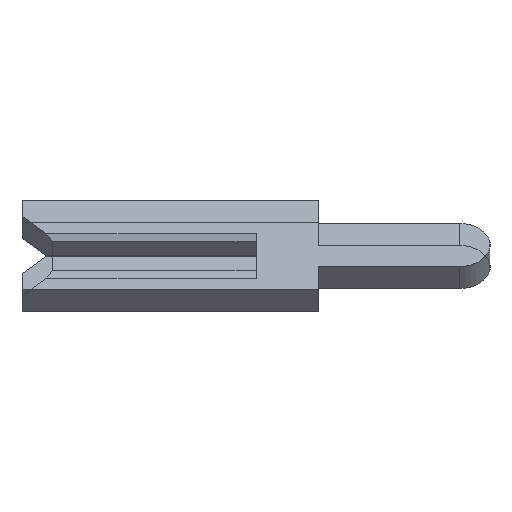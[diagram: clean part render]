
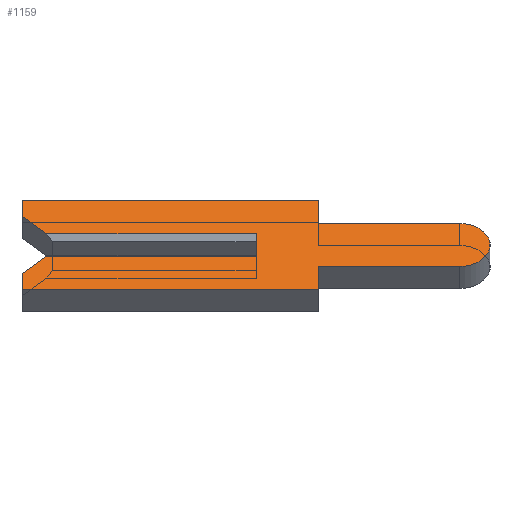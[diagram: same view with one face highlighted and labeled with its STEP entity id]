
A CAD part, left-side view. The second image highlights one B-rep face of the part: STEP entity #1159.
In plain terms, the highlighted face is planar.
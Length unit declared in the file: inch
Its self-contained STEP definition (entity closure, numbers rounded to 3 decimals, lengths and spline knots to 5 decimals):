
#26 = EDGE_CURVE ( 'NONE', #1658, #209, #2182, .T. ) ;
#27 = VERTEX_POINT ( 'NONE', #2498 ) ;
#85 = VECTOR ( 'NONE', #3154, 39.37008 ) ;
#199 = LINE ( 'NONE', #3491, #3130 ) ;
#203 = ORIENTED_EDGE ( 'NONE', *, *, #2566, .F. ) ;
#209 = VERTEX_POINT ( 'NONE', #977 ) ;
#218 = AXIS2_PLACEMENT_3D ( 'NONE', #1717, #3476, #2283 ) ;
#241 = LINE ( 'NONE', #670, #3102 ) ;
#277 = VERTEX_POINT ( 'NONE', #2801 ) ;
#316 = VERTEX_POINT ( 'NONE', #769 ) ;
#359 = VERTEX_POINT ( 'NONE', #442 ) ;
#388 = DIRECTION ( 'NONE',  ( 0., -0.707, 0.707 ) ) ;
#438 = CARTESIAN_POINT ( 'NONE',  ( -0.01, 0.15, 0.026 ) ) ;
#442 = CARTESIAN_POINT ( 'NONE',  ( -0.01, -0.04, 0.04 ) ) ;
#452 = VERTEX_POINT ( 'NONE', #2596 ) ;
#456 = EDGE_CURVE ( 'NONE', #359, #452, #463, .T. ) ;
#463 = LINE ( 'NONE', #2612, #3223 ) ;
#484 = CARTESIAN_POINT ( 'NONE',  ( -0.01, 0., -0.01 ) ) ;
#497 = ORIENTED_EDGE ( 'NONE', *, *, #2163, .F. ) ;
#510 = ORIENTED_EDGE ( 'NONE', *, *, #26, .F. ) ;
#513 = LINE ( 'NONE', #2622, #793 ) ;
#527 = EDGE_CURVE ( 'NONE', #1839, #27, #1992, .T. ) ;
#580 = EDGE_CURVE ( 'NONE', #27, #1653, #199, .T. ) ;
#648 = CARTESIAN_POINT ( 'NONE',  ( -0.01, 0.1305, 0.0065 ) ) ;
#670 = CARTESIAN_POINT ( 'NONE',  ( -0.01, 0.1305, -0.0065 ) ) ;
#762 = EDGE_CURVE ( 'NONE', #3656, #2497, #2223, .T. ) ;
#769 = CARTESIAN_POINT ( 'NONE',  ( -0.01, 0.15, 0.026 ) ) ;
#777 = ORIENTED_EDGE ( 'NONE', *, *, #456, .F. ) ;
#779 = DIRECTION ( 'NONE',  ( 0., 0., -1. ) ) ;
#793 = VECTOR ( 'NONE', #2398, 39.37008 ) ;
#850 = DIRECTION ( 'NONE',  ( 0., -1., 0. ) ) ;
#977 = CARTESIAN_POINT ( 'NONE',  ( -0.01, 0.15, -0.04 ) ) ;
#999 = EDGE_CURVE ( 'NONE', #452, #1839, #513, .T. ) ;
#1031 = CARTESIAN_POINT ( 'NONE',  ( -0.01, -0.04, -0.04 ) ) ;
#1045 = ORIENTED_EDGE ( 'NONE', *, *, #3390, .F. ) ;
#1052 = EDGE_CURVE ( 'NONE', #3469, #3656, #2257, .T. ) ;
#1142 = ORIENTED_EDGE ( 'NONE', *, *, #762, .F. ) ;
#1159 = ADVANCED_FACE ( 'NONE', ( #3205 ), #2961, .F. ) ;
#1189 = VERTEX_POINT ( 'NONE', #3228 ) ;
#1193 = LINE ( 'NONE', #438, #3608 ) ;
#1216 = LINE ( 'NONE', #1435, #3538 ) ;
#1269 = EDGE_CURVE ( 'NONE', #209, #1189, #2440, .T. ) ;
#1344 = VECTOR ( 'NONE', #3193, 39.37008 ) ;
#1412 = LINE ( 'NONE', #2900, #2601 ) ;
#1435 = CARTESIAN_POINT ( 'NONE',  ( -0.01, 0.15, 0.04 ) ) ;
#1442 = DIRECTION ( 'NONE',  ( 0., 0., 1. ) ) ;
#1587 = CARTESIAN_POINT ( 'NONE',  ( -0.01, -0.1305, 0.0195 ) ) ;
#1653 = VERTEX_POINT ( 'NONE', #3701 ) ;
#1658 = VERTEX_POINT ( 'NONE', #1885 ) ;
#1714 = CARTESIAN_POINT ( 'NONE',  ( -0.01, 0.134, 0.01 ) ) ;
#1717 = CARTESIAN_POINT ( 'NONE',  ( -0.01, -0.1305, 0. ) ) ;
#1839 = VERTEX_POINT ( 'NONE', #1587 ) ;
#1885 = CARTESIAN_POINT ( 'NONE',  ( -0.01, -0.04, -0.04 ) ) ;
#1902 = ORIENTED_EDGE ( 'NONE', *, *, #580, .F. ) ;
#1923 = CARTESIAN_POINT ( 'NONE',  ( -0.01, 0.15, -0.04 ) ) ;
#1980 = ORIENTED_EDGE ( 'NONE', *, *, #2767, .F. ) ;
#1992 = CIRCLE ( 'NONE', #218, 0.0195 ) ;
#2134 = EDGE_LOOP ( 'NONE', ( #2554, #1142, #2166, #497, #3259, #510, #203, #1902, #2210, #3501, #777, #1045, #1980, #2694 ) ) ;
#2163 = EDGE_CURVE ( 'NONE', #1189, #3469, #241, .T. ) ;
#2166 = ORIENTED_EDGE ( 'NONE', *, *, #1052, .F. ) ;
#2182 = LINE ( 'NONE', #1923, #85 ) ;
#2210 = ORIENTED_EDGE ( 'NONE', *, *, #527, .F. ) ;
#2223 = LINE ( 'NONE', #3175, #1344 ) ;
#2257 = LINE ( 'NONE', #2661, #2779 ) ;
#2260 = EDGE_CURVE ( 'NONE', #3820, #316, #2956, .T. ) ;
#2283 = DIRECTION ( 'NONE',  ( 0., 0., -1. ) ) ;
#2398 = DIRECTION ( 'NONE',  ( 0., -1., 0. ) ) ;
#2440 = LINE ( 'NONE', #3241, #3406 ) ;
#2497 = VERTEX_POINT ( 'NONE', #2530 ) ;
#2498 = CARTESIAN_POINT ( 'NONE',  ( -0.01, -0.1305, -0.0195 ) ) ;
#2506 = DIRECTION ( 'NONE',  ( 0., 0., -1. ) ) ;
#2530 = CARTESIAN_POINT ( 'NONE',  ( -0.01, 0., 0.01 ) ) ;
#2554 = ORIENTED_EDGE ( 'NONE', *, *, #3644, .T. ) ;
#2566 = EDGE_CURVE ( 'NONE', #1653, #1658, #3379, .T. ) ;
#2596 = CARTESIAN_POINT ( 'NONE',  ( -0.01, -0.04, 0.0195 ) ) ;
#2601 = VECTOR ( 'NONE', #3528, 39.37008 ) ;
#2612 = CARTESIAN_POINT ( 'NONE',  ( -0.01, -0.04, 0.04 ) ) ;
#2622 = CARTESIAN_POINT ( 'NONE',  ( -0.01, -0.04, 0.0195 ) ) ;
#2661 = CARTESIAN_POINT ( 'NONE',  ( -0.01, -0.1305, -0.01 ) ) ;
#2694 = ORIENTED_EDGE ( 'NONE', *, *, #2260, .F. ) ;
#2767 = EDGE_CURVE ( 'NONE', #316, #277, #1193, .T. ) ;
#2779 = VECTOR ( 'NONE', #850, 39.37008 ) ;
#2801 = CARTESIAN_POINT ( 'NONE',  ( -0.01, 0.15, 0.04 ) ) ;
#2900 = CARTESIAN_POINT ( 'NONE',  ( -0.01, 0.15, 0.01 ) ) ;
#2916 = DIRECTION ( 'NONE',  ( 1., 0., 0. ) ) ;
#2956 = LINE ( 'NONE', #648, #3337 ) ;
#2961 = PLANE ( 'NONE',  #3495 ) ;
#2975 = DIRECTION ( 'NONE',  ( 0., 0., -1. ) ) ;
#3102 = VECTOR ( 'NONE', #388, 39.37008 ) ;
#3130 = VECTOR ( 'NONE', #3218, 39.37008 ) ;
#3154 = DIRECTION ( 'NONE',  ( 0., 1., 0. ) ) ;
#3162 = DIRECTION ( 'NONE',  ( 0., 0., 1. ) ) ;
#3173 = DIRECTION ( 'NONE',  ( 0., 0.707, 0.707 ) ) ;
#3175 = CARTESIAN_POINT ( 'NONE',  ( -0.01, 0., 0.0065 ) ) ;
#3189 = DIRECTION ( 'NONE',  ( 0., -1., 0. ) ) ;
#3193 = DIRECTION ( 'NONE',  ( 0., 0., 1. ) ) ;
#3205 = FACE_OUTER_BOUND ( 'NONE', #2134, .T. ) ;
#3218 = DIRECTION ( 'NONE',  ( 0., 1., 0. ) ) ;
#3223 = VECTOR ( 'NONE', #779, 39.37008 ) ;
#3228 = CARTESIAN_POINT ( 'NONE',  ( -0.01, 0.15, -0.026 ) ) ;
#3241 = CARTESIAN_POINT ( 'NONE',  ( -0.01, 0.15, -0.026 ) ) ;
#3259 = ORIENTED_EDGE ( 'NONE', *, *, #1269, .F. ) ;
#3268 = CARTESIAN_POINT ( 'NONE',  ( -0.01, -0.1305, 0. ) ) ;
#3337 = VECTOR ( 'NONE', #3173, 39.37008 ) ;
#3379 = LINE ( 'NONE', #1031, #3594 ) ;
#3390 = EDGE_CURVE ( 'NONE', #277, #359, #1216, .T. ) ;
#3406 = VECTOR ( 'NONE', #1442, 39.37008 ) ;
#3469 = VERTEX_POINT ( 'NONE', #3513 ) ;
#3476 = DIRECTION ( 'NONE',  ( 1., 0., 0. ) ) ;
#3491 = CARTESIAN_POINT ( 'NONE',  ( -0.01, -0.04, -0.0195 ) ) ;
#3495 = AXIS2_PLACEMENT_3D ( 'NONE', #3268, #2916, #2975 ) ;
#3501 = ORIENTED_EDGE ( 'NONE', *, *, #999, .F. ) ;
#3513 = CARTESIAN_POINT ( 'NONE',  ( -0.01, 0.134, -0.01 ) ) ;
#3528 = DIRECTION ( 'NONE',  ( 0., -1., 0. ) ) ;
#3538 = VECTOR ( 'NONE', #3189, 39.37008 ) ;
#3594 = VECTOR ( 'NONE', #2506, 39.37008 ) ;
#3608 = VECTOR ( 'NONE', #3162, 39.37008 ) ;
#3644 = EDGE_CURVE ( 'NONE', #3820, #2497, #1412, .T. ) ;
#3656 = VERTEX_POINT ( 'NONE', #484 ) ;
#3701 = CARTESIAN_POINT ( 'NONE',  ( -0.01, -0.04, -0.0195 ) ) ;
#3820 = VERTEX_POINT ( 'NONE', #1714 ) ;
